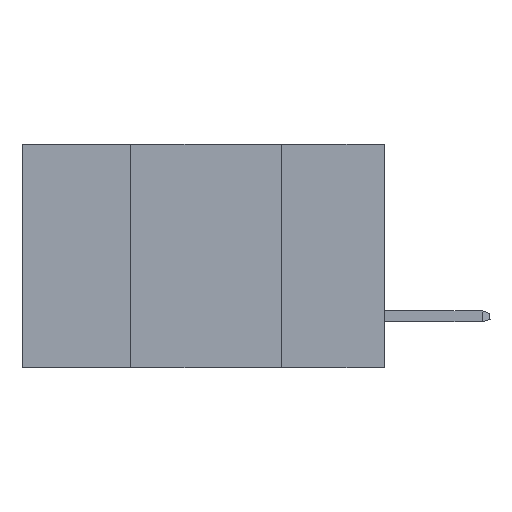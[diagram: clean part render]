
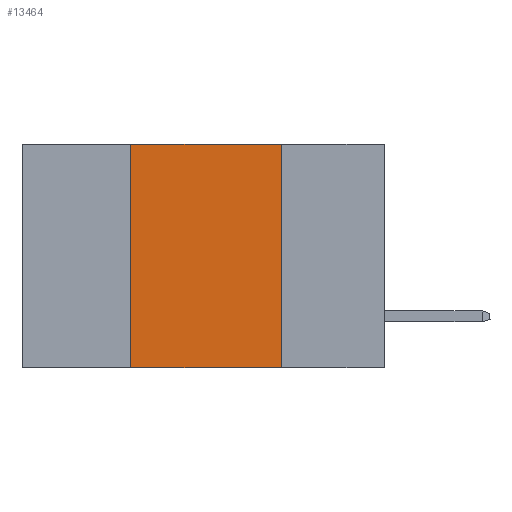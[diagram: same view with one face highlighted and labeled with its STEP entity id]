
A CAD part, left-side view. The second image highlights one B-rep face of the part: STEP entity #13464.
In plain terms, the highlighted planar face has unit normal (-1, 0, 0).
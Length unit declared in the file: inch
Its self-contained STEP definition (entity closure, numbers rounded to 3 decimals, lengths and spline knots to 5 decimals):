
#759 = LINE ( 'NONE', #10324, #12239 ) ;
#1166 = VERTEX_POINT ( 'NONE', #5361 ) ;
#1345 = EDGE_LOOP ( 'NONE', ( #5946, #10663, #3177, #14607 ) ) ;
#1974 = VERTEX_POINT ( 'NONE', #14797 ) ;
#2815 = CARTESIAN_POINT ( 'NONE',  ( 0., 0.6, 0. ) ) ;
#3177 = ORIENTED_EDGE ( 'NONE', *, *, #12668, .F. ) ;
#3589 = AXIS2_PLACEMENT_3D ( 'NONE', #5747, #12250, #8186 ) ;
#4308 = DIRECTION ( 'NONE',  ( 0., -1., 0. ) ) ;
#4730 = EDGE_CURVE ( 'NONE', #1974, #1166, #759, .T. ) ;
#4846 = EDGE_CURVE ( 'NONE', #12144, #1974, #12607, .T. ) ;
#4996 = LINE ( 'NONE', #5596, #16089 ) ;
#5361 = CARTESIAN_POINT ( 'NONE',  ( 0., 0.17, -0.37 ) ) ;
#5596 = CARTESIAN_POINT ( 'NONE',  ( 0., 0.42, 0. ) ) ;
#5747 = CARTESIAN_POINT ( 'NONE',  ( 0., 0.6, 0. ) ) ;
#5946 = ORIENTED_EDGE ( 'NONE', *, *, #4730, .F. ) ;
#6276 = EDGE_CURVE ( 'NONE', #11428, #1166, #13003, .T. ) ;
#6754 = VECTOR ( 'NONE', #4308, 39.37008 ) ;
#6778 = CARTESIAN_POINT ( 'NONE',  ( 0., 0.42, 0. ) ) ;
#7376 = DIRECTION ( 'NONE',  ( 0., 0., 1. ) ) ;
#8186 = DIRECTION ( 'NONE',  ( 0., 0., -1. ) ) ;
#9607 = VECTOR ( 'NONE', #12733, 39.37008 ) ;
#10027 = CARTESIAN_POINT ( 'NONE',  ( 0., 0.6, -0.37 ) ) ;
#10273 = DIRECTION ( 'NONE',  ( 0., 0., -1. ) ) ;
#10324 = CARTESIAN_POINT ( 'NONE',  ( 0., 0.17, 0. ) ) ;
#10663 = ORIENTED_EDGE ( 'NONE', *, *, #4846, .F. ) ;
#11428 = VERTEX_POINT ( 'NONE', #13781 ) ;
#12068 = FACE_OUTER_BOUND ( 'NONE', #1345, .T. ) ;
#12073 = PLANE ( 'NONE',  #3589 ) ;
#12144 = VERTEX_POINT ( 'NONE', #6778 ) ;
#12239 = VECTOR ( 'NONE', #10273, 39.37008 ) ;
#12250 = DIRECTION ( 'NONE',  ( 1., 0., 0. ) ) ;
#12607 = LINE ( 'NONE', #2815, #6754 ) ;
#12668 = EDGE_CURVE ( 'NONE', #11428, #12144, #4996, .T. ) ;
#12733 = DIRECTION ( 'NONE',  ( 0., -1., 0. ) ) ;
#13003 = LINE ( 'NONE', #10027, #9607 ) ;
#13464 = ADVANCED_FACE ( 'NONE', ( #12068 ), #12073, .F. ) ;
#13781 = CARTESIAN_POINT ( 'NONE',  ( 0., 0.42, -0.37 ) ) ;
#14607 = ORIENTED_EDGE ( 'NONE', *, *, #6276, .T. ) ;
#14797 = CARTESIAN_POINT ( 'NONE',  ( 0., 0.17, 0. ) ) ;
#16089 = VECTOR ( 'NONE', #7376, 39.37008 ) ;
